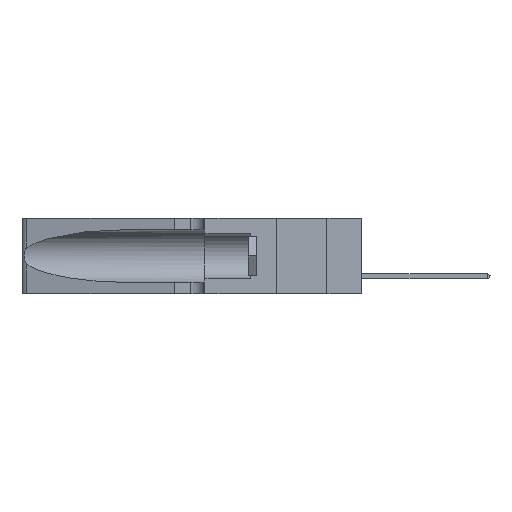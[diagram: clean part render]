
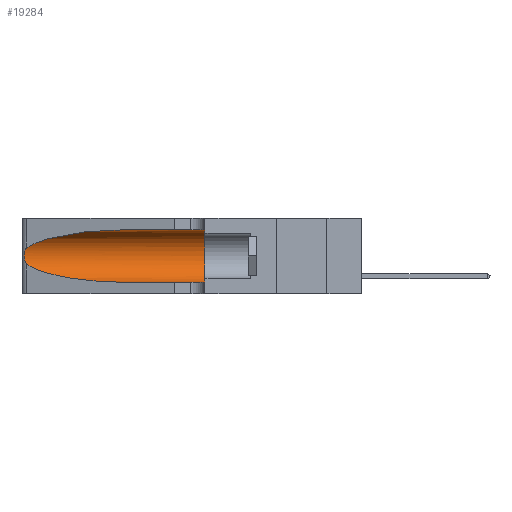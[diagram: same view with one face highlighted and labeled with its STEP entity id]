
A CAD part, left-side view. The second image highlights one B-rep face of the part: STEP entity #19284.
In plain terms, the highlighted cylindrical face has radius 3.308 mm (diameter 6.617 mm), a partial arc.
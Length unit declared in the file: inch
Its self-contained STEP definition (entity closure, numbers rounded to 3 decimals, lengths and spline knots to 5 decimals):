
#3330 =( BOUNDED_CURVE ( )  B_SPLINE_CURVE ( 3, ( #23371, #34937, #50803, #27248 ),
 .UNSPECIFIED., .F., .F. ) 
 B_SPLINE_CURVE_WITH_KNOTS ( ( 4, 4 ),
 ( 1.5708, 2.84003 ),
 .UNSPECIFIED. ) 
 CURVE ( )  GEOMETRIC_REPRESENTATION_ITEM ( )  RATIONAL_B_SPLINE_CURVE ( ( 1., 0.87, 0.87, 1. ) ) 
 REPRESENTATION_ITEM ( '' )  );
#3723 = VERTEX_POINT ( 'NONE', #27440 ) ;
#3987 = VERTEX_POINT ( 'NONE', #41051 ) ;
#4301 = CARTESIAN_POINT ( 'NONE',  ( 0.25555, 1.22994, 0.2215 ) ) ;
#4597 = ORIENTED_EDGE ( 'NONE', *, *, #24719, .T. ) ;
#4919 = ORIENTED_EDGE ( 'NONE', *, *, #13257, .T. ) ;
#5402 = EDGE_CURVE ( 'NONE', #3987, #24739, #27151, .T. ) ;
#5406 = DIRECTION ( 'NONE',  ( 0., 0., 1. ) ) ;
#5997 = EDGE_CURVE ( 'NONE', #32406, #24739, #9333, .T. ) ;
#6406 = CARTESIAN_POINT ( 'NONE',  ( 0.25487, 1.22718, 0.14631 ) ) ;
#8073 = DIRECTION ( 'NONE',  ( 0., 1., 0. ) ) ;
#8302 = CARTESIAN_POINT ( 'NONE',  ( 0.1305, 0.35, 0.31525 ) ) ;
#8958 = CARTESIAN_POINT ( 'NONE',  ( 0.25787, 1.23484, 0.2124 ) ) ;
#9333 = CIRCLE ( 'NONE', #17931, 0.13025 ) ;
#10012 = CARTESIAN_POINT ( 'NONE',  ( 0.26017, 1.23833, 0.17102 ) ) ;
#11398 = AXIS2_PLACEMENT_3D ( 'NONE', #42669, #18713, #34273 ) ;
#12971 = CARTESIAN_POINT ( 'NONE',  ( 0.25854, 1.2359, 0.20912 ) ) ;
#13257 = EDGE_CURVE ( 'NONE', #20589, #3987, #35175, .T. ) ;
#13541 = CARTESIAN_POINT ( 'NONE',  ( 0.1305, 0.35, 0.05475 ) ) ;
#15513 = ORIENTED_EDGE ( 'NONE', *, *, #5997, .F. ) ;
#16355 = CARTESIAN_POINT ( 'NONE',  ( 0.2373, 1.15595, 0.08982 ) ) ;
#17150 = LINE ( 'NONE', #21320, #18512 ) ;
#17931 = AXIS2_PLACEMENT_3D ( 'NONE', #19860, #8073, #5406 ) ;
#18512 = VECTOR ( 'NONE', #49301, 39.37008 ) ;
#18713 = DIRECTION ( 'NONE',  ( 0., -1., 0. ) ) ;
#19228 = CARTESIAN_POINT ( 'NONE',  ( 0.25856, 1.23593, 0.16098 ) ) ;
#19284 = ADVANCED_FACE ( 'NONE', ( #39349 ), #26779, .F. ) ;
#19860 = CARTESIAN_POINT ( 'NONE',  ( 0.1305, 0.35, 0.185 ) ) ;
#20550 = CARTESIAN_POINT ( 'NONE',  ( 0.1305, 0.72297, 0.05475 ) ) ;
#20589 = VERTEX_POINT ( 'NONE', #6406 ) ;
#21320 = CARTESIAN_POINT ( 'NONE',  ( 0.1305, 1.61858, 0.31525 ) ) ;
#22461 = DIRECTION ( 'NONE',  ( 0., -1., 0. ) ) ;
#22821 = EDGE_CURVE ( 'NONE', #3723, #20589, #29626, .T. ) ;
#22882 = CARTESIAN_POINT ( 'NONE',  ( 0.25789, 1.23486, 0.15765 ) ) ;
#23371 = CARTESIAN_POINT ( 'NONE',  ( 0.1305, 0.72297, 0.31525 ) ) ;
#24719 = EDGE_CURVE ( 'NONE', #38214, #3723, #3330, .T. ) ;
#24739 = VERTEX_POINT ( 'NONE', #13541 ) ;
#26560 = CARTESIAN_POINT ( 'NONE',  ( 0.26018, 1.23835, 0.19895 ) ) ;
#26779 = CYLINDRICAL_SURFACE ( 'NONE', #11398, 0.13025 ) ;
#27151 = LINE ( 'NONE', #38034, #40270 ) ;
#27248 = CARTESIAN_POINT ( 'NONE',  ( 0.25487, 1.22718, 0.22369 ) ) ;
#27440 = CARTESIAN_POINT ( 'NONE',  ( 0.25487, 1.22718, 0.22369 ) ) ;
#27979 = CARTESIAN_POINT ( 'NONE',  ( 0.25639, 1.23186, 0.15144 ) ) ;
#28497 = ORIENTED_EDGE ( 'NONE', *, *, #5402, .T. ) ;
#29626 = B_SPLINE_CURVE_WITH_KNOTS ( 'NONE', 3,
 ( #44671, #4301, #45693, #8958, #12971, #26560, #38659, #37887, #10012, #19228, #22882, #27979, #40040, #44152 ),
 .UNSPECIFIED., .F., .F.,
 ( 4, 2, 2, 2, 2, 2, 4 ),
 ( 0., 0.00027, 0.00053, 0.00107, 0.0016, 0.00187, 0.00214 ),
 .UNSPECIFIED. ) ;
#30971 = EDGE_LOOP ( 'NONE', ( #4597, #40394, #4919, #28497, #15513, #32323 ) ) ;
#32323 = ORIENTED_EDGE ( 'NONE', *, *, #37959, .F. ) ;
#32406 = VERTEX_POINT ( 'NONE', #8302 ) ;
#33347 = CARTESIAN_POINT ( 'NONE',  ( 0.1305, 0.72297, 0.31525 ) ) ;
#34273 = DIRECTION ( 'NONE',  ( 0., 0., -1. ) ) ;
#34937 = CARTESIAN_POINT ( 'NONE',  ( 0.18966, 0.96281, 0.31525 ) ) ;
#35175 =( BOUNDED_CURVE ( )  B_SPLINE_CURVE ( 3, ( #48381, #16355, #36520, #20550 ),
 .UNSPECIFIED., .F., .T. ) 
 B_SPLINE_CURVE_WITH_KNOTS ( ( 4, 4 ),
 ( 3.44316, 4.71239 ),
 .UNSPECIFIED. ) 
 CURVE ( )  GEOMETRIC_REPRESENTATION_ITEM ( )  RATIONAL_B_SPLINE_CURVE ( ( 1., 0.87, 0.87, 1. ) ) 
 REPRESENTATION_ITEM ( '' )  );
#36520 = CARTESIAN_POINT ( 'NONE',  ( 0.18966, 0.96281, 0.05475 ) ) ;
#37887 = CARTESIAN_POINT ( 'NONE',  ( 0.26075, 1.23896, 0.178 ) ) ;
#37959 = EDGE_CURVE ( 'NONE', #38214, #32406, #17150, .T. ) ;
#38034 = CARTESIAN_POINT ( 'NONE',  ( 0.1305, 1.61858, 0.05475 ) ) ;
#38214 = VERTEX_POINT ( 'NONE', #33347 ) ;
#38659 = CARTESIAN_POINT ( 'NONE',  ( 0.26075, 1.23896, 0.19203 ) ) ;
#39349 = FACE_OUTER_BOUND ( 'NONE', #30971, .T. ) ;
#40040 = CARTESIAN_POINT ( 'NONE',  ( 0.25555, 1.22993, 0.14849 ) ) ;
#40270 = VECTOR ( 'NONE', #22461, 39.37008 ) ;
#40394 = ORIENTED_EDGE ( 'NONE', *, *, #22821, .T. ) ;
#41051 = CARTESIAN_POINT ( 'NONE',  ( 0.1305, 0.72297, 0.05475 ) ) ;
#42669 = CARTESIAN_POINT ( 'NONE',  ( 0.1305, 1.61858, 0.185 ) ) ;
#44152 = CARTESIAN_POINT ( 'NONE',  ( 0.25487, 1.22718, 0.14631 ) ) ;
#44671 = CARTESIAN_POINT ( 'NONE',  ( 0.25487, 1.22718, 0.22369 ) ) ;
#45693 = CARTESIAN_POINT ( 'NONE',  ( 0.25639, 1.23184, 0.21858 ) ) ;
#48381 = CARTESIAN_POINT ( 'NONE',  ( 0.25487, 1.22718, 0.14631 ) ) ;
#49301 = DIRECTION ( 'NONE',  ( 0., -1., 0. ) ) ;
#50803 = CARTESIAN_POINT ( 'NONE',  ( 0.2373, 1.15595, 0.28018 ) ) ;
